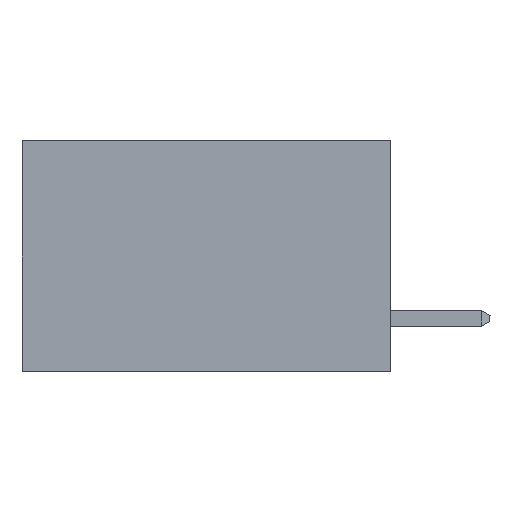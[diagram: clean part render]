
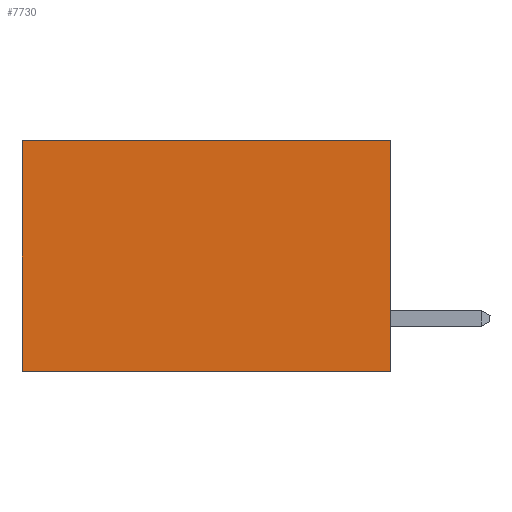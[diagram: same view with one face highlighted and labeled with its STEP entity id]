
A CAD part, left-side view. The second image highlights one B-rep face of the part: STEP entity #7730.
In plain terms, the highlighted planar face has unit normal (-1, 0, 0).
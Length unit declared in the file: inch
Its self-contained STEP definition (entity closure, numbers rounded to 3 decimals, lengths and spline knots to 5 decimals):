
#371 = DIRECTION ( 'NONE',  ( 0., 0., -1. ) ) ;
#432 = CARTESIAN_POINT ( 'NONE',  ( 0.277, 0., -0.37 ) ) ;
#2866 = VECTOR ( 'NONE', #9092, 39.37008 ) ;
#3133 = LINE ( 'NONE', #6805, #22537 ) ;
#3393 = EDGE_LOOP ( 'NONE', ( #5373, #7268, #19178, #20386 ) ) ;
#3439 = CARTESIAN_POINT ( 'NONE',  ( 0.277, 0.59, -0.37 ) ) ;
#3664 = LINE ( 'NONE', #432, #8640 ) ;
#4662 = CARTESIAN_POINT ( 'NONE',  ( 0.277, 0.59, 0. ) ) ;
#4745 = VERTEX_POINT ( 'NONE', #22261 ) ;
#5261 = DIRECTION ( 'NONE',  ( 0., 1., 0. ) ) ;
#5373 = ORIENTED_EDGE ( 'NONE', *, *, #20364, .T. ) ;
#6805 = CARTESIAN_POINT ( 'NONE',  ( 0.277, 0., -0.37 ) ) ;
#7268 = ORIENTED_EDGE ( 'NONE', *, *, #20999, .F. ) ;
#7433 = EDGE_CURVE ( 'NONE', #20609, #21366, #3664, .T. ) ;
#7730 = ADVANCED_FACE ( 'NONE', ( #15883 ), #18951, .F. ) ;
#8640 = VECTOR ( 'NONE', #371, 39.37008 ) ;
#9092 = DIRECTION ( 'NONE',  ( 0., 0., -1. ) ) ;
#10357 = VERTEX_POINT ( 'NONE', #4662 ) ;
#12370 = DIRECTION ( 'NONE',  ( 0., 1., 0. ) ) ;
#12875 = LINE ( 'NONE', #22075, #22370 ) ;
#13373 = LINE ( 'NONE', #3439, #2866 ) ;
#15124 = EDGE_CURVE ( 'NONE', #20609, #10357, #12875, .T. ) ;
#15573 = CARTESIAN_POINT ( 'NONE',  ( 0.277, 0., 0. ) ) ;
#15883 = FACE_OUTER_BOUND ( 'NONE', #3393, .T. ) ;
#17137 = AXIS2_PLACEMENT_3D ( 'NONE', #18253, #18223, #18195 ) ;
#18195 = DIRECTION ( 'NONE',  ( 0., 0., -1. ) ) ;
#18223 = DIRECTION ( 'NONE',  ( 1., 0., 0. ) ) ;
#18253 = CARTESIAN_POINT ( 'NONE',  ( 0.277, 0., -0.37 ) ) ;
#18951 = PLANE ( 'NONE',  #17137 ) ;
#19005 = CARTESIAN_POINT ( 'NONE',  ( 0.277, 0., -0.37 ) ) ;
#19178 = ORIENTED_EDGE ( 'NONE', *, *, #7433, .F. ) ;
#20364 = EDGE_CURVE ( 'NONE', #10357, #4745, #13373, .T. ) ;
#20386 = ORIENTED_EDGE ( 'NONE', *, *, #15124, .T. ) ;
#20609 = VERTEX_POINT ( 'NONE', #15573 ) ;
#20999 = EDGE_CURVE ( 'NONE', #21366, #4745, #3133, .T. ) ;
#21366 = VERTEX_POINT ( 'NONE', #19005 ) ;
#22075 = CARTESIAN_POINT ( 'NONE',  ( 0.277, 0., 0. ) ) ;
#22261 = CARTESIAN_POINT ( 'NONE',  ( 0.277, 0.59, -0.37 ) ) ;
#22370 = VECTOR ( 'NONE', #5261, 39.37008 ) ;
#22537 = VECTOR ( 'NONE', #12370, 39.37008 ) ;
